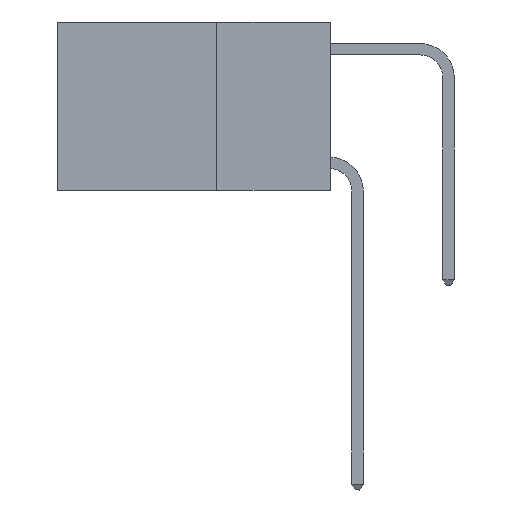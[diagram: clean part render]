
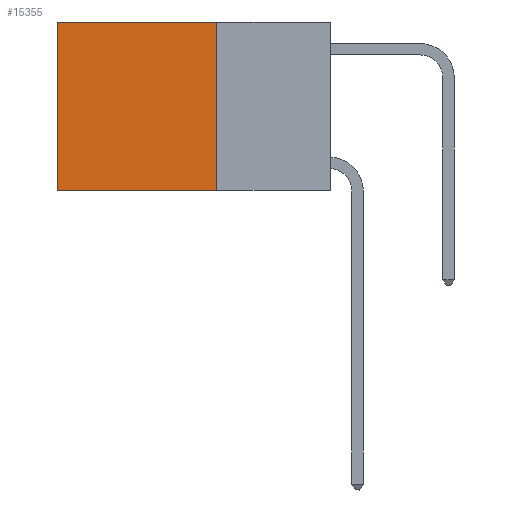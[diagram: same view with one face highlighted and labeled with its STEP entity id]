
A CAD part, left-side view. The second image highlights one B-rep face of the part: STEP entity #15355.
In plain terms, the highlighted planar face has unit normal (-1, 0, 0).
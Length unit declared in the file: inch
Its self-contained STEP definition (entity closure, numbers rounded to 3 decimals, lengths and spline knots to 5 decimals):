
#182 = LINE ( 'NONE', #14234, #3940 ) ;
#2079 = ORIENTED_EDGE ( 'NONE', *, *, #15463, .T. ) ;
#2098 = EDGE_CURVE ( 'NONE', #13058, #10755, #7733, .T. ) ;
#2356 = EDGE_CURVE ( 'NONE', #12936, #13172, #11683, .T. ) ;
#2447 = CARTESIAN_POINT ( 'NONE',  ( 0.2625, 0.25, -0.37 ) ) ;
#2800 = DIRECTION ( 'NONE',  ( 0., 0., -1. ) ) ;
#3074 = DIRECTION ( 'NONE',  ( 0., 0., -1. ) ) ;
#3118 = VECTOR ( 'NONE', #12355, 39.37008 ) ;
#3217 = VECTOR ( 'NONE', #17186, 39.37008 ) ;
#3767 = CARTESIAN_POINT ( 'NONE',  ( 0.2625, 0.25, 0. ) ) ;
#3940 = VECTOR ( 'NONE', #3074, 39.37008 ) ;
#7155 = ORIENTED_EDGE ( 'NONE', *, *, #2356, .T. ) ;
#7304 = AXIS2_PLACEMENT_3D ( 'NONE', #10725, #12363, #2800 ) ;
#7665 = CARTESIAN_POINT ( 'NONE',  ( 0.2625, 0.25, 0. ) ) ;
#7733 = LINE ( 'NONE', #11904, #15659 ) ;
#10718 = CARTESIAN_POINT ( 'NONE',  ( 0.2625, 0.25, 0. ) ) ;
#10725 = CARTESIAN_POINT ( 'NONE',  ( 0.2625, 0.25, 0. ) ) ;
#10755 = VERTEX_POINT ( 'NONE', #15120 ) ;
#10785 = EDGE_LOOP ( 'NONE', ( #2079, #16294, #13617, #7155 ) ) ;
#11344 = EDGE_CURVE ( 'NONE', #12936, #13058, #15782, .T. ) ;
#11683 = LINE ( 'NONE', #7665, #3217 ) ;
#11904 = CARTESIAN_POINT ( 'NONE',  ( 0.2625, 0.25, -0.37 ) ) ;
#12355 = DIRECTION ( 'NONE',  ( 0., 0., -1. ) ) ;
#12363 = DIRECTION ( 'NONE',  ( 1., 0., 0. ) ) ;
#12936 = VERTEX_POINT ( 'NONE', #3767 ) ;
#13058 = VERTEX_POINT ( 'NONE', #2447 ) ;
#13172 = VERTEX_POINT ( 'NONE', #19997 ) ;
#13617 = ORIENTED_EDGE ( 'NONE', *, *, #11344, .F. ) ;
#14234 = CARTESIAN_POINT ( 'NONE',  ( 0.2625, 0.6, 0. ) ) ;
#15025 = DIRECTION ( 'NONE',  ( 0., 1., 0. ) ) ;
#15120 = CARTESIAN_POINT ( 'NONE',  ( 0.2625, 0.6, -0.37 ) ) ;
#15355 = ADVANCED_FACE ( 'NONE', ( #18515 ), #20062, .F. ) ;
#15463 = EDGE_CURVE ( 'NONE', #13172, #10755, #182, .T. ) ;
#15659 = VECTOR ( 'NONE', #15025, 39.37008 ) ;
#15782 = LINE ( 'NONE', #10718, #3118 ) ;
#16294 = ORIENTED_EDGE ( 'NONE', *, *, #2098, .F. ) ;
#17186 = DIRECTION ( 'NONE',  ( 0., 1., 0. ) ) ;
#18515 = FACE_OUTER_BOUND ( 'NONE', #10785, .T. ) ;
#19997 = CARTESIAN_POINT ( 'NONE',  ( 0.2625, 0.6, 0. ) ) ;
#20062 = PLANE ( 'NONE',  #7304 ) ;
